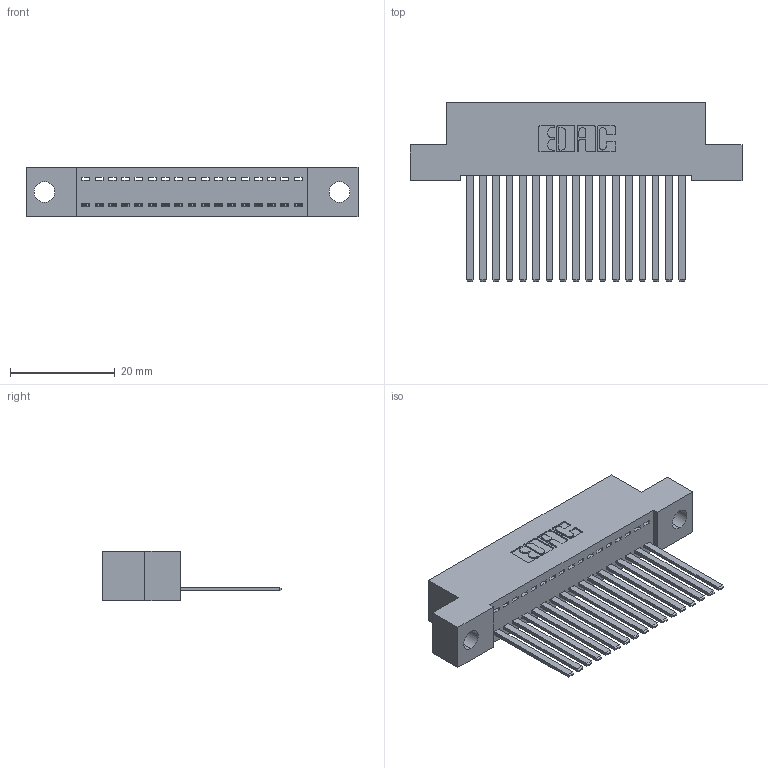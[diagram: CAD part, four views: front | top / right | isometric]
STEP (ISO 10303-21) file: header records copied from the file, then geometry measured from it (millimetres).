
FILE_DESCRIPTION (( 'STEP AP203' ), '1' );
FILE_NAME ('342-017-544-104.STEP', '2019-10-01T19:31:54', ( '' ), ( '' ), 'SwSTEP 2.0', 'SolidWorks 2016', '' );
FILE_SCHEMA (( 'CONFIG_CONTROL_DESIGN' ));
Length unit declared in the file: inch
Products named in the file (3): 342 Part_.156 TH; 345-292-001_345-293-144; 342-017-544-104
Assembly tree (18 placements, depth 2):
  342-017-544-104
    342 Part_.156 TH
    345-292-001_345-293-144  x17
Bounding box: 63.5 x 34.3 x 9.4 mm (x, y, z)
Volume: 5585.5 mm3; surface area: 8114.3 mm2
Topology: 18 solids, 18 shells, 994 faces, 2985 edges, 1966 vertices
Faces by surface type: plane 712, cylinder 282
Entity records: 13313 total; most frequent: CARTESIAN_POINT 2305, ORIENTED_EDGE 2258, DIRECTION 1991, EDGE_CURVE 1129, VECTOR 1005, LINE 1005, VERTEX_POINT 750, AXIS2_PLACEMENT_3D 493
